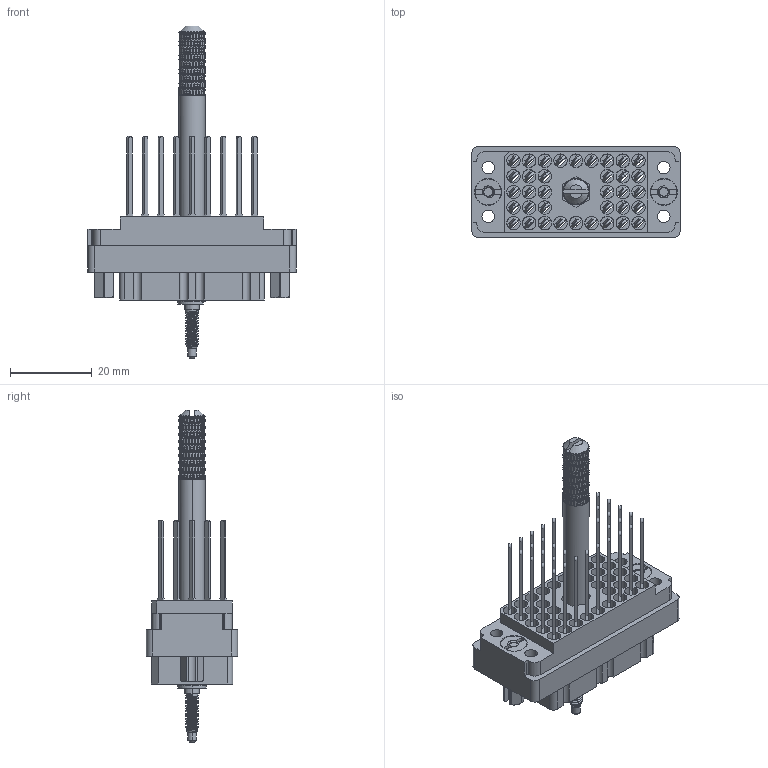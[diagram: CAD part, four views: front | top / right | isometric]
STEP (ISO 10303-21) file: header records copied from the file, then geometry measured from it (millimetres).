
FILE_DESCRIPTION (( 'STEP AP203' ), '1' );
FILE_NAME ('519-036-542-401.STEP', '2020-09-09T22:44:56', ( '' ), ( '' ), 'SwSTEP 2.0', 'SolidWorks 2020', '' );
FILE_SCHEMA (( 'CONFIG_CONTROL_DESIGN' ));
Length unit declared in the file: inch
Products named in the file (11): 516-292-001_542 Contact; Actuating Screw Assy 038-056; 519-036-542-401; 516-253-035-100; 516-221-038-102_038; 516-221-038-102_039; 516-251-035-100; 516-250-038-111; 519 Receptacle Insulator_036; 516-252-021-102_038; 516-253-138-107
Assembly tree (47 placements, depth 3):
  519-036-542-401
    519 Receptacle Insulator_036
    516-292-001_542 Contact  x36
    Actuating Screw Assy 038-056
      516-251-035-100
      516-253-035-100  x2
      516-253-138-107
      516-250-038-111
    516-252-021-102_038  x2
    516-221-038-102_038
    516-221-038-102_039
Bounding box: 50.8 x 22.25 x 81.03 mm (x, y, z)
Volume: 15285.6 mm3; surface area: 25128.9 mm2
Topology: 46 solids, 46 shells, 5006 faces, 13425 edges, 8528 vertices
Faces by surface type: plane 2246, cylinder 1458, bspline 1250, cone 52
Entity records: 107664 total; most frequent: CARTESIAN_POINT 59167, ORIENTED_EDGE 12078, DIRECTION 7042, EDGE_CURVE 6039, VERTEX_POINT 3630, EDGE_LOOP 2565, FACE_OUTER_BOUND 2449, ADVANCED_FACE 2449
